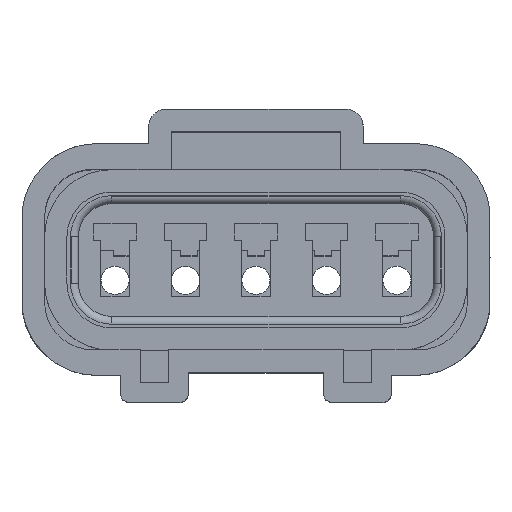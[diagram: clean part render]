
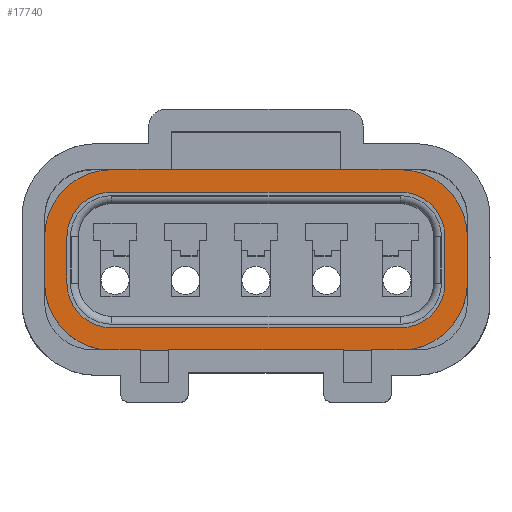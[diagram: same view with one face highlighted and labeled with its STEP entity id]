
A CAD part, top view. The second image highlights one B-rep face of the part: STEP entity #17740.
In plain terms, the highlighted face is planar.
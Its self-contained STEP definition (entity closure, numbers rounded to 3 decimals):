
#326 = VECTOR ( 'NONE', #20091, 1000. ) ;
#697 = ORIENTED_EDGE ( 'NONE', *, *, #7271, .T. ) ;
#756 = CARTESIAN_POINT ( 'NONE',  ( -5.12, 3.2, 0. ) ) ;
#833 = VECTOR ( 'NONE', #10036, 1000. ) ;
#941 = CARTESIAN_POINT ( 'NONE',  ( -7.5, 0.82, 0. ) ) ;
#1204 = CARTESIAN_POINT ( 'NONE',  ( 6.705, -0.82, 0. ) ) ;
#1365 = DIRECTION ( 'NONE',  ( 1., 0., 0. ) ) ;
#2060 = CARTESIAN_POINT ( 'NONE',  ( -5.12, -3.2, 0. ) ) ;
#2266 = EDGE_CURVE ( 'NONE', #5387, #15124, #18564, .T. ) ;
#2365 = LINE ( 'NONE', #8795, #326 ) ;
#2424 = DIRECTION ( 'NONE',  ( 0., 0., 1. ) ) ;
#2636 = DIRECTION ( 'NONE',  ( 1., 0., 0. ) ) ;
#2649 = AXIS2_PLACEMENT_3D ( 'NONE', #20145, #2424, #3866 ) ;
#2671 = DIRECTION ( 'NONE',  ( 0., -1., 0. ) ) ;
#2814 = VERTEX_POINT ( 'NONE', #756 ) ;
#2883 = EDGE_CURVE ( 'NONE', #15016, #5102, #11488, .T. ) ;
#2971 = DIRECTION ( 'NONE',  ( 1., 0., 0. ) ) ;
#3141 = LINE ( 'NONE', #10952, #20579 ) ;
#3261 = DIRECTION ( 'NONE',  ( 1., 0., 0. ) ) ;
#3277 = DIRECTION ( 'NONE',  ( 0., 0., 1. ) ) ;
#3343 = ORIENTED_EDGE ( 'NONE', *, *, #2883, .F. ) ;
#3445 = CARTESIAN_POINT ( 'NONE',  ( 5.12, -3.2, 0. ) ) ;
#3585 = LINE ( 'NONE', #6878, #833 ) ;
#3701 = CIRCLE ( 'NONE', #18224, 1.585 ) ;
#3866 = DIRECTION ( 'NONE',  ( 1., 0., 0. ) ) ;
#3929 = VERTEX_POINT ( 'NONE', #11550 ) ;
#4141 = EDGE_CURVE ( 'NONE', #14615, #9895, #2365, .T. ) ;
#4211 = CARTESIAN_POINT ( 'NONE',  ( -5.12, -0.82, 0. ) ) ;
#4326 = ORIENTED_EDGE ( 'NONE', *, *, #4141, .T. ) ;
#4356 = CARTESIAN_POINT ( 'NONE',  ( 5.12, -0.82, 0. ) ) ;
#4919 = PLANE ( 'NONE',  #17967 ) ;
#5093 = DIRECTION ( 'NONE',  ( 1., 0., 0. ) ) ;
#5102 = VERTEX_POINT ( 'NONE', #2060 ) ;
#5225 = ORIENTED_EDGE ( 'NONE', *, *, #11625, .F. ) ;
#5306 = EDGE_CURVE ( 'NONE', #18692, #19036, #15449, .T. ) ;
#5357 = AXIS2_PLACEMENT_3D ( 'NONE', #18615, #20183, #20394 ) ;
#5387 = VERTEX_POINT ( 'NONE', #6876 ) ;
#5794 = VERTEX_POINT ( 'NONE', #941 ) ;
#5836 = CARTESIAN_POINT ( 'NONE',  ( -6.705, 0.82, 0. ) ) ;
#5893 = ORIENTED_EDGE ( 'NONE', *, *, #6508, .F. ) ;
#6015 = VECTOR ( 'NONE', #6155, 1000. ) ;
#6029 = ORIENTED_EDGE ( 'NONE', *, *, #14857, .T. ) ;
#6030 = DIRECTION ( 'NONE',  ( 1., 0., 0. ) ) ;
#6155 = DIRECTION ( 'NONE',  ( 1., 0., 0. ) ) ;
#6418 = FACE_OUTER_BOUND ( 'NONE', #10753, .T. ) ;
#6508 = EDGE_CURVE ( 'NONE', #5102, #17770, #12675, .T. ) ;
#6522 = FACE_BOUND ( 'NONE', #17025, .T. ) ;
#6571 = CARTESIAN_POINT ( 'NONE',  ( -5.12, 2.405, 0. ) ) ;
#6849 = LINE ( 'NONE', #8527, #10390 ) ;
#6876 = CARTESIAN_POINT ( 'NONE',  ( 7.5, 0.82, 0. ) ) ;
#6878 = CARTESIAN_POINT ( 'NONE',  ( 7.5, -0.82, 0. ) ) ;
#7198 = LINE ( 'NONE', #16376, #18150 ) ;
#7199 = ORIENTED_EDGE ( 'NONE', *, *, #5306, .T. ) ;
#7271 = EDGE_CURVE ( 'NONE', #14763, #14615, #14443, .T. ) ;
#7327 = VECTOR ( 'NONE', #3261, 1000. ) ;
#7859 = CARTESIAN_POINT ( 'NONE',  ( 5.12, 0.82, 0. ) ) ;
#8179 = ORIENTED_EDGE ( 'NONE', *, *, #9570, .T. ) ;
#8527 = CARTESIAN_POINT ( 'NONE',  ( -7.5, 0.82, 0. ) ) ;
#8795 = CARTESIAN_POINT ( 'NONE',  ( 6.705, -0.82, 0. ) ) ;
#9139 = DIRECTION ( 'NONE',  ( 0., 0., 1. ) ) ;
#9261 = ORIENTED_EDGE ( 'NONE', *, *, #11678, .F. ) ;
#9419 = LINE ( 'NONE', #6571, #6015 ) ;
#9526 = CARTESIAN_POINT ( 'NONE',  ( 5.12, 2.405, 0. ) ) ;
#9570 = EDGE_CURVE ( 'NONE', #3929, #18692, #19543, .T. ) ;
#9598 = EDGE_CURVE ( 'NONE', #17770, #10330, #11130, .T. ) ;
#9895 = VERTEX_POINT ( 'NONE', #18617 ) ;
#9929 = VERTEX_POINT ( 'NONE', #9526 ) ;
#9975 = EDGE_CURVE ( 'NONE', #19036, #20082, #3701, .T. ) ;
#10036 = DIRECTION ( 'NONE',  ( 0., 1., 0. ) ) ;
#10156 = ORIENTED_EDGE ( 'NONE', *, *, #16070, .T. ) ;
#10330 = VERTEX_POINT ( 'NONE', #20065 ) ;
#10390 = VECTOR ( 'NONE', #13295, 1000. ) ;
#10431 = AXIS2_PLACEMENT_3D ( 'NONE', #18519, #13876, #12179 ) ;
#10590 = DIRECTION ( 'NONE',  ( 0., 0., 1. ) ) ;
#10753 = EDGE_LOOP ( 'NONE', ( #9261, #16910, #18335, #16062, #15703, #5893, #3343, #5225 ) ) ;
#10930 = DIRECTION ( 'NONE',  ( 1., 0., 0. ) ) ;
#10952 = CARTESIAN_POINT ( 'NONE',  ( -5.12, 3.2, 0. ) ) ;
#11084 = CARTESIAN_POINT ( 'NONE',  ( -5.12, -3.2, 0. ) ) ;
#11130 = CIRCLE ( 'NONE', #14522, 2.38 ) ;
#11361 = CARTESIAN_POINT ( 'NONE',  ( -5.12, 2.405, 0. ) ) ;
#11488 = CIRCLE ( 'NONE', #15206, 2.38 ) ;
#11550 = CARTESIAN_POINT ( 'NONE',  ( -5.12, 2.405, 0. ) ) ;
#11625 = EDGE_CURVE ( 'NONE', #5794, #15016, #6849, .T. ) ;
#11678 = EDGE_CURVE ( 'NONE', #2814, #5794, #11742, .T. ) ;
#11742 = CIRCLE ( 'NONE', #2649, 2.38 ) ;
#11841 = CARTESIAN_POINT ( 'NONE',  ( -6.705, 0.82, 0. ) ) ;
#12179 = DIRECTION ( 'NONE',  ( 1., 0., 0. ) ) ;
#12209 = EDGE_CURVE ( 'NONE', #3929, #9929, #9419, .T. ) ;
#12370 = DIRECTION ( 'NONE',  ( 0., 0., 1. ) ) ;
#12675 = LINE ( 'NONE', #11084, #7327 ) ;
#12854 = CARTESIAN_POINT ( 'NONE',  ( 5.12, -0.82, 0. ) ) ;
#12882 = ORIENTED_EDGE ( 'NONE', *, *, #9975, .T. ) ;
#13194 = EDGE_CURVE ( 'NONE', #2814, #15124, #3141, .T. ) ;
#13295 = DIRECTION ( 'NONE',  ( 0., -1., 0. ) ) ;
#13876 = DIRECTION ( 'NONE',  ( 0., 0., 1. ) ) ;
#14443 = CIRCLE ( 'NONE', #20850, 1.585 ) ;
#14522 = AXIS2_PLACEMENT_3D ( 'NONE', #4356, #10590, #15453 ) ;
#14615 = VERTEX_POINT ( 'NONE', #1204 ) ;
#14662 = ORIENTED_EDGE ( 'NONE', *, *, #12209, .F. ) ;
#14763 = VERTEX_POINT ( 'NONE', #15989 ) ;
#14857 = EDGE_CURVE ( 'NONE', #20082, #14763, #7198, .T. ) ;
#15016 = VERTEX_POINT ( 'NONE', #17652 ) ;
#15124 = VERTEX_POINT ( 'NONE', #18056 ) ;
#15206 = AXIS2_PLACEMENT_3D ( 'NONE', #4211, #17092, #2636 ) ;
#15449 = LINE ( 'NONE', #5836, #20099 ) ;
#15453 = DIRECTION ( 'NONE',  ( 1., 0., 0. ) ) ;
#15703 = ORIENTED_EDGE ( 'NONE', *, *, #9598, .F. ) ;
#15989 = CARTESIAN_POINT ( 'NONE',  ( 5.12, -2.405, 0. ) ) ;
#16062 = ORIENTED_EDGE ( 'NONE', *, *, #19772, .F. ) ;
#16070 = EDGE_CURVE ( 'NONE', #9895, #9929, #17140, .T. ) ;
#16175 = CARTESIAN_POINT ( 'NONE',  ( -5.12, -0.82, 0. ) ) ;
#16376 = CARTESIAN_POINT ( 'NONE',  ( -5.12, -2.405, 0. ) ) ;
#16881 = CARTESIAN_POINT ( 'NONE',  ( -5.12, -2.405, 0. ) ) ;
#16910 = ORIENTED_EDGE ( 'NONE', *, *, #13194, .T. ) ;
#17025 = EDGE_LOOP ( 'NONE', ( #14662, #8179, #7199, #12882, #6029, #697, #4326, #10156 ) ) ;
#17092 = DIRECTION ( 'NONE',  ( 0., 0., 1. ) ) ;
#17140 = CIRCLE ( 'NONE', #5357, 1.585 ) ;
#17652 = CARTESIAN_POINT ( 'NONE',  ( -7.5, -0.82, 0. ) ) ;
#17740 = ADVANCED_FACE ( 'NONE', ( #6418, #6522 ), #4919, .T. ) ;
#17770 = VERTEX_POINT ( 'NONE', #3445 ) ;
#17889 = AXIS2_PLACEMENT_3D ( 'NONE', #7859, #12370, #2971 ) ;
#17967 = AXIS2_PLACEMENT_3D ( 'NONE', #11361, #19199, #19499 ) ;
#18056 = CARTESIAN_POINT ( 'NONE',  ( 5.12, 3.2, 0. ) ) ;
#18150 = VECTOR ( 'NONE', #5093, 1000. ) ;
#18224 = AXIS2_PLACEMENT_3D ( 'NONE', #16175, #3277, #6030 ) ;
#18268 = CARTESIAN_POINT ( 'NONE',  ( -6.705, -0.82, 0. ) ) ;
#18335 = ORIENTED_EDGE ( 'NONE', *, *, #2266, .F. ) ;
#18519 = CARTESIAN_POINT ( 'NONE',  ( -5.12, 0.82, 0. ) ) ;
#18564 = CIRCLE ( 'NONE', #17889, 2.38 ) ;
#18615 = CARTESIAN_POINT ( 'NONE',  ( 5.12, 0.82, 0. ) ) ;
#18617 = CARTESIAN_POINT ( 'NONE',  ( 6.705, 0.82, 0. ) ) ;
#18692 = VERTEX_POINT ( 'NONE', #11841 ) ;
#19036 = VERTEX_POINT ( 'NONE', #18268 ) ;
#19199 = DIRECTION ( 'NONE',  ( 0., 0., -1. ) ) ;
#19499 = DIRECTION ( 'NONE',  ( 0., 1., 0. ) ) ;
#19543 = CIRCLE ( 'NONE', #10431, 1.585 ) ;
#19772 = EDGE_CURVE ( 'NONE', #10330, #5387, #3585, .T. ) ;
#20065 = CARTESIAN_POINT ( 'NONE',  ( 7.5, -0.82, 0. ) ) ;
#20082 = VERTEX_POINT ( 'NONE', #16881 ) ;
#20091 = DIRECTION ( 'NONE',  ( 0., 1., 0. ) ) ;
#20099 = VECTOR ( 'NONE', #2671, 1000. ) ;
#20145 = CARTESIAN_POINT ( 'NONE',  ( -5.12, 0.82, 0. ) ) ;
#20183 = DIRECTION ( 'NONE',  ( 0., 0., 1. ) ) ;
#20394 = DIRECTION ( 'NONE',  ( 1., 0., 0. ) ) ;
#20579 = VECTOR ( 'NONE', #1365, 1000. ) ;
#20850 = AXIS2_PLACEMENT_3D ( 'NONE', #12854, #9139, #10930 ) ;
